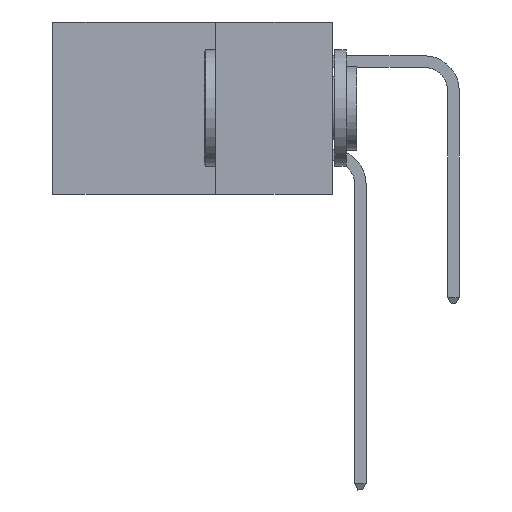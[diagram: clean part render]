
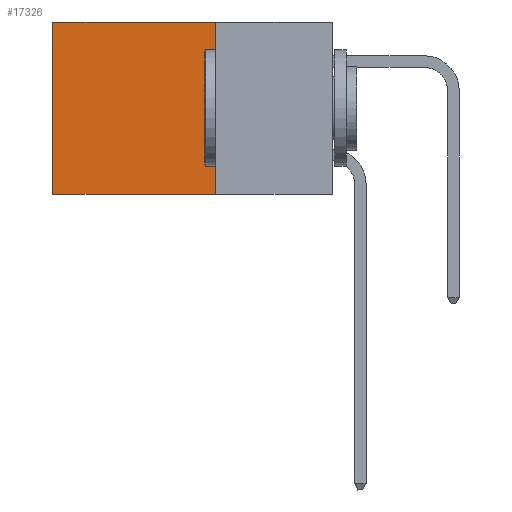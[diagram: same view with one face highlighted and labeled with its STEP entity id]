
A CAD part, left-side view. The second image highlights one B-rep face of the part: STEP entity #17326.
In plain terms, the highlighted planar face has unit normal (-1, 0, 0).
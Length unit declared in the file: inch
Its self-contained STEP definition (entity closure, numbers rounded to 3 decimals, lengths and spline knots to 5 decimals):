
#314 = EDGE_CURVE ( 'NONE', #6451, #11695, #18624, .T. ) ;
#1592 = DIRECTION ( 'NONE',  ( 0., 0., -1. ) ) ;
#3203 = DIRECTION ( 'NONE',  ( 0., 1., 0. ) ) ;
#3633 = EDGE_LOOP ( 'NONE', ( #16388, #20504, #16228, #15887 ) ) ;
#4131 = CARTESIAN_POINT ( 'NONE',  ( 0.2615, 0.25, -0.37 ) ) ;
#4620 = DIRECTION ( 'NONE',  ( 0., 0., -1. ) ) ;
#4926 = VECTOR ( 'NONE', #1592, 39.37008 ) ;
#5583 = CARTESIAN_POINT ( 'NONE',  ( 0.2615, 0.25, 0. ) ) ;
#5996 = LINE ( 'NONE', #19102, #15930 ) ;
#6451 = VERTEX_POINT ( 'NONE', #24232 ) ;
#8045 = VECTOR ( 'NONE', #8672, 39.37008 ) ;
#8094 = LINE ( 'NONE', #17738, #22438 ) ;
#8672 = DIRECTION ( 'NONE',  ( 0., 1., 0. ) ) ;
#11596 = CARTESIAN_POINT ( 'NONE',  ( 0.2615, 0.25, -0.37 ) ) ;
#11695 = VERTEX_POINT ( 'NONE', #15869 ) ;
#12106 = AXIS2_PLACEMENT_3D ( 'NONE', #16397, #16487, #4620 ) ;
#14495 = PLANE ( 'NONE',  #12106 ) ;
#15467 = LINE ( 'NONE', #11596, #4926 ) ;
#15707 = FACE_OUTER_BOUND ( 'NONE', #3633, .T. ) ;
#15869 = CARTESIAN_POINT ( 'NONE',  ( 0.2615, 0.6, 0. ) ) ;
#15887 = ORIENTED_EDGE ( 'NONE', *, *, #314, .T. ) ;
#15930 = VECTOR ( 'NONE', #3203, 39.37008 ) ;
#16228 = ORIENTED_EDGE ( 'NONE', *, *, #21184, .F. ) ;
#16388 = ORIENTED_EDGE ( 'NONE', *, *, #19961, .T. ) ;
#16397 = CARTESIAN_POINT ( 'NONE',  ( 0.2615, 0.25, -0.37 ) ) ;
#16487 = DIRECTION ( 'NONE',  ( 1., 0., 0. ) ) ;
#17194 = VERTEX_POINT ( 'NONE', #17978 ) ;
#17326 = ADVANCED_FACE ( 'NONE', ( #15707 ), #14495, .F. ) ;
#17738 = CARTESIAN_POINT ( 'NONE',  ( 0.2615, 0.6, -0.37 ) ) ;
#17978 = CARTESIAN_POINT ( 'NONE',  ( 0.2615, 0.6, -0.37 ) ) ;
#18488 = VERTEX_POINT ( 'NONE', #4131 ) ;
#18624 = LINE ( 'NONE', #5583, #8045 ) ;
#18881 = EDGE_CURVE ( 'NONE', #18488, #17194, #5996, .T. ) ;
#19102 = CARTESIAN_POINT ( 'NONE',  ( 0.2615, 0.25, -0.37 ) ) ;
#19720 = DIRECTION ( 'NONE',  ( 0., 0., -1. ) ) ;
#19961 = EDGE_CURVE ( 'NONE', #11695, #17194, #8094, .T. ) ;
#20504 = ORIENTED_EDGE ( 'NONE', *, *, #18881, .F. ) ;
#21184 = EDGE_CURVE ( 'NONE', #6451, #18488, #15467, .T. ) ;
#22438 = VECTOR ( 'NONE', #19720, 39.37008 ) ;
#24232 = CARTESIAN_POINT ( 'NONE',  ( 0.2615, 0.25, 0. ) ) ;
